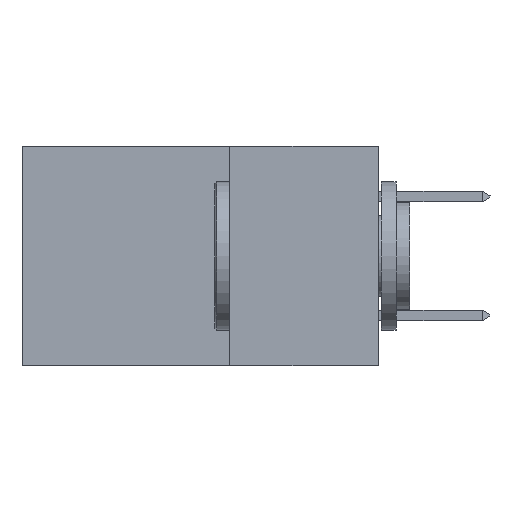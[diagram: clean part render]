
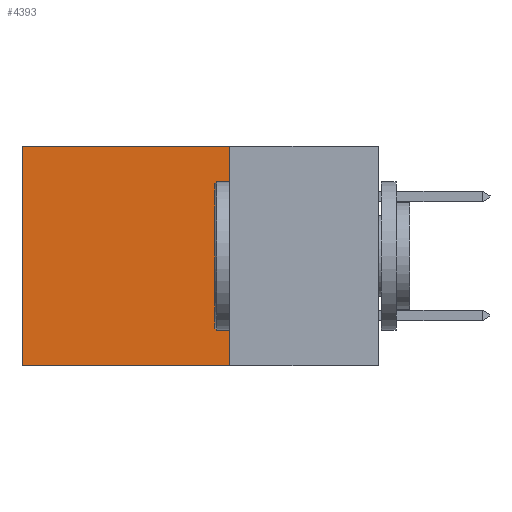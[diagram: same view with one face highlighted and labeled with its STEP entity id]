
A CAD part, left-side view. The second image highlights one B-rep face of the part: STEP entity #4393.
In plain terms, the highlighted planar face has unit normal (-1, 0, 0).
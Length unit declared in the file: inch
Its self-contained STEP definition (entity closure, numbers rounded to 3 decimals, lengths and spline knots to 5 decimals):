
#19 = LINE ( 'NONE', #4704, #2015 ) ;
#123 = VECTOR ( 'NONE', #3692, 39.37008 ) ;
#208 = ORIENTED_EDGE ( 'NONE', *, *, #11604, .T. ) ;
#913 = LINE ( 'NONE', #3716, #2605 ) ;
#1600 = EDGE_CURVE ( 'NONE', #8889, #1744, #3140, .T. ) ;
#1744 = VERTEX_POINT ( 'NONE', #4259 ) ;
#2015 = VECTOR ( 'NONE', #10409, 39.37008 ) ;
#2381 = PLANE ( 'NONE',  #7078 ) ;
#2605 = VECTOR ( 'NONE', #11072, 39.37008 ) ;
#3140 = LINE ( 'NONE', #10602, #7385 ) ;
#3335 = CARTESIAN_POINT ( 'NONE',  ( 0.2615, 0.25, -0.37 ) ) ;
#3448 = CARTESIAN_POINT ( 'NONE',  ( 0.2615, 0.6, -0.37 ) ) ;
#3692 = DIRECTION ( 'NONE',  ( 0., 1., 0. ) ) ;
#3716 = CARTESIAN_POINT ( 'NONE',  ( 0.2615, 0.25, -0.37 ) ) ;
#3864 = CARTESIAN_POINT ( 'NONE',  ( 0.2615, 0.25, -0.37 ) ) ;
#4176 = DIRECTION ( 'NONE',  ( 0., 1., 0. ) ) ;
#4246 = DIRECTION ( 'NONE',  ( 0., 0., -1. ) ) ;
#4259 = CARTESIAN_POINT ( 'NONE',  ( 0.2615, 0.6, 0. ) ) ;
#4393 = ADVANCED_FACE ( 'NONE', ( #9785 ), #2381, .F. ) ;
#4704 = CARTESIAN_POINT ( 'NONE',  ( 0.2615, 0.6, -0.37 ) ) ;
#4785 = LINE ( 'NONE', #3864, #123 ) ;
#5506 = CARTESIAN_POINT ( 'NONE',  ( 0.2615, 0.25, 0. ) ) ;
#5895 = EDGE_CURVE ( 'NONE', #11299, #6130, #4785, .T. ) ;
#6130 = VERTEX_POINT ( 'NONE', #3448 ) ;
#6934 = ORIENTED_EDGE ( 'NONE', *, *, #10649, .F. ) ;
#7078 = AXIS2_PLACEMENT_3D ( 'NONE', #3335, #9726, #4246 ) ;
#7385 = VECTOR ( 'NONE', #4176, 39.37008 ) ;
#7672 = ORIENTED_EDGE ( 'NONE', *, *, #1600, .T. ) ;
#8139 = CARTESIAN_POINT ( 'NONE',  ( 0.2615, 0.25, -0.37 ) ) ;
#8889 = VERTEX_POINT ( 'NONE', #5506 ) ;
#9726 = DIRECTION ( 'NONE',  ( 1., 0., 0. ) ) ;
#9785 = FACE_OUTER_BOUND ( 'NONE', #10836, .T. ) ;
#9860 = ORIENTED_EDGE ( 'NONE', *, *, #5895, .F. ) ;
#10409 = DIRECTION ( 'NONE',  ( 0., 0., -1. ) ) ;
#10602 = CARTESIAN_POINT ( 'NONE',  ( 0.2615, 0.25, 0. ) ) ;
#10649 = EDGE_CURVE ( 'NONE', #8889, #11299, #913, .T. ) ;
#10836 = EDGE_LOOP ( 'NONE', ( #208, #9860, #6934, #7672 ) ) ;
#11072 = DIRECTION ( 'NONE',  ( 0., 0., -1. ) ) ;
#11299 = VERTEX_POINT ( 'NONE', #8139 ) ;
#11604 = EDGE_CURVE ( 'NONE', #1744, #6130, #19, .T. ) ;
